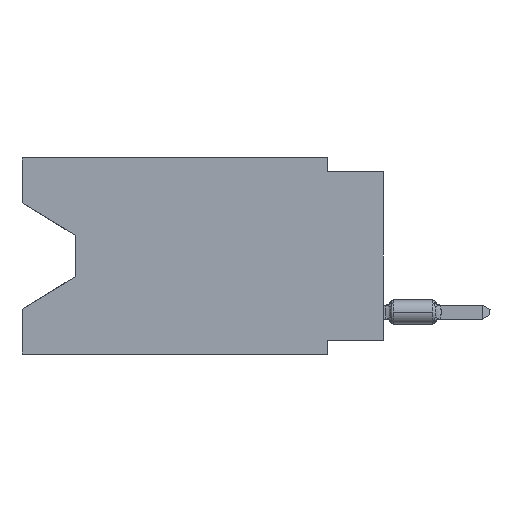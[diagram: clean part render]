
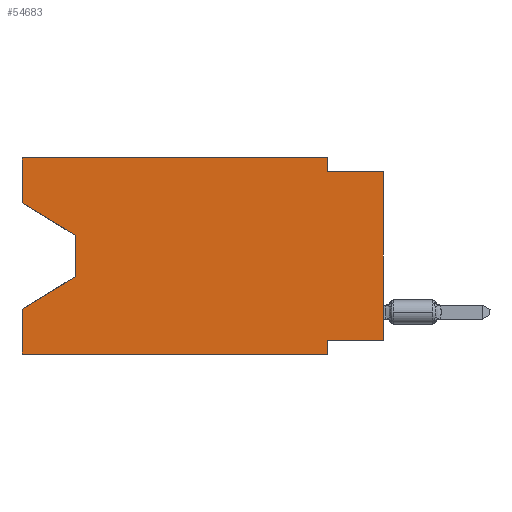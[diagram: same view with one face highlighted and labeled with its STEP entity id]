
A CAD part, left-side view. The second image highlights one B-rep face of the part: STEP entity #54683.
In plain terms, the highlighted planar face has unit normal (-1, 0, 0).
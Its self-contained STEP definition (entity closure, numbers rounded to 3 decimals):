
#1032 = LINE ( 'NONE', #47154, #6158 ) ;
#2473 = ORIENTED_EDGE ( 'NONE', *, *, #41863, .F. ) ;
#2692 = LINE ( 'NONE', #48148, #18936 ) ;
#3468 = DIRECTION ( 'NONE',  ( 0., 0.855, -0.519 ) ) ;
#3657 = VECTOR ( 'NONE', #5107, 1000. ) ;
#3898 = ORIENTED_EDGE ( 'NONE', *, *, #46364, .F. ) ;
#5107 = DIRECTION ( 'NONE',  ( 0., -1., 0. ) ) ;
#5523 = CARTESIAN_POINT ( 'NONE',  ( 0., 13.97, -3.505 ) ) ;
#6158 = VECTOR ( 'NONE', #12374, 1000. ) ;
#6332 = ORIENTED_EDGE ( 'NONE', *, *, #54403, .T. ) ;
#6449 = PLANE ( 'NONE',  #42221 ) ;
#7025 = VECTOR ( 'NONE', #3468, 1000. ) ;
#7098 = CARTESIAN_POINT ( 'NONE',  ( 0., 16.383, 0. ) ) ;
#7303 = VECTOR ( 'NONE', #35751, 1000. ) ;
#7980 = VERTEX_POINT ( 'NONE', #48398 ) ;
#9012 = EDGE_CURVE ( 'NONE', #53456, #7980, #51166, .T. ) ;
#9450 = CARTESIAN_POINT ( 'NONE',  ( 0., 13.97, -3.505 ) ) ;
#10168 = VECTOR ( 'NONE', #20459, 1000. ) ;
#10460 = CARTESIAN_POINT ( 'NONE',  ( 0., 0., -0.635 ) ) ;
#10876 = DIRECTION ( 'NONE',  ( 0., 0., -1. ) ) ;
#10908 = ORIENTED_EDGE ( 'NONE', *, *, #46325, .F. ) ;
#11795 = ORIENTED_EDGE ( 'NONE', *, *, #9012, .F. ) ;
#12214 = LINE ( 'NONE', #47636, #44869 ) ;
#12374 = DIRECTION ( 'NONE',  ( 0., 0., -1. ) ) ;
#14429 = CARTESIAN_POINT ( 'NONE',  ( 0., 16.383, 0. ) ) ;
#15396 = LINE ( 'NONE', #15717, #7303 ) ;
#15717 = CARTESIAN_POINT ( 'NONE',  ( 0., 16.383, -2.038 ) ) ;
#16139 = VERTEX_POINT ( 'NONE', #45086 ) ;
#16487 = DIRECTION ( 'NONE',  ( 1., 0., 0. ) ) ;
#16823 = FACE_OUTER_BOUND ( 'NONE', #55844, .T. ) ;
#17625 = VECTOR ( 'NONE', #19781, 1000. ) ;
#18191 = DIRECTION ( 'NONE',  ( 0., 0., 1. ) ) ;
#18777 = CARTESIAN_POINT ( 'NONE',  ( 0., 2.54, -8.89 ) ) ;
#18936 = VECTOR ( 'NONE', #43452, 1000. ) ;
#19781 = DIRECTION ( 'NONE',  ( 0., 0., 1. ) ) ;
#20459 = DIRECTION ( 'NONE',  ( 0., -1., 0. ) ) ;
#20671 = CARTESIAN_POINT ( 'NONE',  ( 0., 16.383, -2.038 ) ) ;
#21447 = DIRECTION ( 'NONE',  ( 0., 0., 1. ) ) ;
#23640 = VERTEX_POINT ( 'NONE', #49653 ) ;
#24120 = LINE ( 'NONE', #18777, #65043 ) ;
#25001 = CARTESIAN_POINT ( 'NONE',  ( 0., 2.54, -8.89 ) ) ;
#25936 = EDGE_CURVE ( 'NONE', #33144, #63152, #24120, .T. ) ;
#27601 = CARTESIAN_POINT ( 'NONE',  ( 0., 2.54, 0. ) ) ;
#27667 = EDGE_CURVE ( 'NONE', #34230, #23640, #61969, .T. ) ;
#28769 = ORIENTED_EDGE ( 'NONE', *, *, #56320, .F. ) ;
#28787 = EDGE_CURVE ( 'NONE', #7980, #38036, #12214, .T. ) ;
#30033 = VERTEX_POINT ( 'NONE', #32940 ) ;
#30350 = ORIENTED_EDGE ( 'NONE', *, *, #57453, .T. ) ;
#31560 = EDGE_CURVE ( 'NONE', #38299, #63152, #40535, .T. ) ;
#32940 = CARTESIAN_POINT ( 'NONE',  ( 0., 16.383, -6.852 ) ) ;
#33144 = VERTEX_POINT ( 'NONE', #34599 ) ;
#34230 = VERTEX_POINT ( 'NONE', #9450 ) ;
#34599 = CARTESIAN_POINT ( 'NONE',  ( 0., 2.54, -8.255 ) ) ;
#35751 = DIRECTION ( 'NONE',  ( 0., -0.855, -0.519 ) ) ;
#37878 = VECTOR ( 'NONE', #21447, 1000. ) ;
#38036 = VERTEX_POINT ( 'NONE', #27601 ) ;
#38299 = VERTEX_POINT ( 'NONE', #61425 ) ;
#39124 = DIRECTION ( 'NONE',  ( 0., 0., -1. ) ) ;
#40128 = CARTESIAN_POINT ( 'NONE',  ( 0., 0., -0.635 ) ) ;
#40535 = LINE ( 'NONE', #41849, #3657 ) ;
#41849 = CARTESIAN_POINT ( 'NONE',  ( 0., 16.383, -8.89 ) ) ;
#41863 = EDGE_CURVE ( 'NONE', #16139, #33144, #2692, .T. ) ;
#42221 = AXIS2_PLACEMENT_3D ( 'NONE', #7098, #16487, #59103 ) ;
#43452 = DIRECTION ( 'NONE',  ( 0., 1., 0. ) ) ;
#43604 = DIRECTION ( 'NONE',  ( 0., -1., 0. ) ) ;
#43618 = ORIENTED_EDGE ( 'NONE', *, *, #51106, .T. ) ;
#44650 = ORIENTED_EDGE ( 'NONE', *, *, #31560, .T. ) ;
#44826 = LINE ( 'NONE', #40128, #10168 ) ;
#44869 = VECTOR ( 'NONE', #43604, 1000. ) ;
#45086 = CARTESIAN_POINT ( 'NONE',  ( 0., 0., -8.255 ) ) ;
#45389 = CARTESIAN_POINT ( 'NONE',  ( 0., 2.54, -0.635 ) ) ;
#46325 = EDGE_CURVE ( 'NONE', #38299, #30033, #65863, .T. ) ;
#46364 = EDGE_CURVE ( 'NONE', #53750, #58334, #44826, .T. ) ;
#47147 = CARTESIAN_POINT ( 'NONE',  ( 0., 16.383, 0. ) ) ;
#47154 = CARTESIAN_POINT ( 'NONE',  ( 0., 2.54, 0. ) ) ;
#47448 = VECTOR ( 'NONE', #18191, 1000. ) ;
#47636 = CARTESIAN_POINT ( 'NONE',  ( 0., 16.383, 0. ) ) ;
#48148 = CARTESIAN_POINT ( 'NONE',  ( 0., 0., -8.255 ) ) ;
#48398 = CARTESIAN_POINT ( 'NONE',  ( 0., 16.383, 0. ) ) ;
#48605 = CARTESIAN_POINT ( 'NONE',  ( 0., 13.97, -5.385 ) ) ;
#49269 = LINE ( 'NONE', #48605, #7025 ) ;
#49653 = CARTESIAN_POINT ( 'NONE',  ( 0., 13.97, -5.385 ) ) ;
#51106 = EDGE_CURVE ( 'NONE', #16139, #58334, #58909, .T. ) ;
#51166 = LINE ( 'NONE', #47147, #37878 ) ;
#53456 = VERTEX_POINT ( 'NONE', #20671 ) ;
#53750 = VERTEX_POINT ( 'NONE', #45389 ) ;
#54403 = EDGE_CURVE ( 'NONE', #23640, #30033, #49269, .T. ) ;
#54566 = CARTESIAN_POINT ( 'NONE',  ( 0., 0., 0. ) ) ;
#54683 = ADVANCED_FACE ( 'NONE', ( #16823 ), #6449, .F. ) ;
#55844 = EDGE_LOOP ( 'NONE', ( #30350, #56303, #6332, #10908, #44650, #57267, #2473, #43618, #3898, #28769, #58602, #11795 ) ) ;
#56303 = ORIENTED_EDGE ( 'NONE', *, *, #27667, .T. ) ;
#56320 = EDGE_CURVE ( 'NONE', #38036, #53750, #1032, .T. ) ;
#57267 = ORIENTED_EDGE ( 'NONE', *, *, #25936, .F. ) ;
#57453 = EDGE_CURVE ( 'NONE', #53456, #34230, #15396, .T. ) ;
#58334 = VERTEX_POINT ( 'NONE', #10460 ) ;
#58602 = ORIENTED_EDGE ( 'NONE', *, *, #28787, .F. ) ;
#58909 = LINE ( 'NONE', #54566, #47448 ) ;
#59103 = DIRECTION ( 'NONE',  ( 0., 0., -1. ) ) ;
#61425 = CARTESIAN_POINT ( 'NONE',  ( 0., 16.383, -8.89 ) ) ;
#61969 = LINE ( 'NONE', #5523, #63082 ) ;
#63082 = VECTOR ( 'NONE', #10876, 1000. ) ;
#63152 = VERTEX_POINT ( 'NONE', #25001 ) ;
#65043 = VECTOR ( 'NONE', #39124, 1000. ) ;
#65863 = LINE ( 'NONE', #14429, #17625 ) ;
